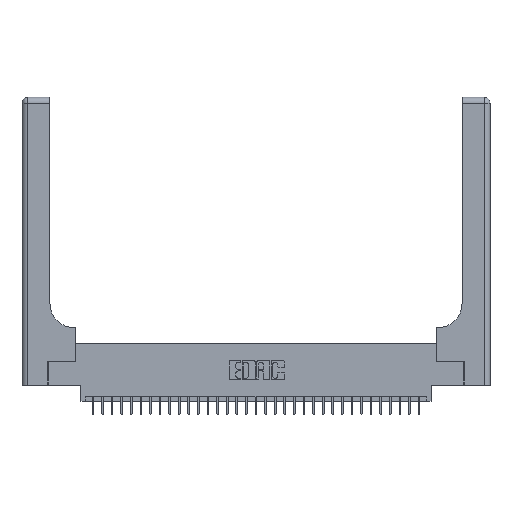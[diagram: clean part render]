
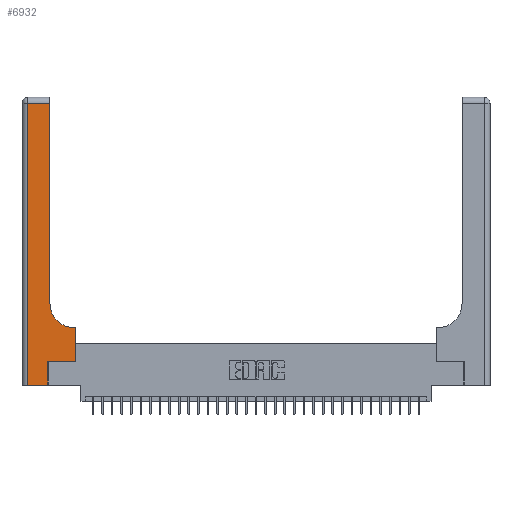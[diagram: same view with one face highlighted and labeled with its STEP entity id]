
A CAD part, top view. The second image highlights one B-rep face of the part: STEP entity #6932.
In plain terms, the highlighted planar face has unit normal (0, 0, 1).
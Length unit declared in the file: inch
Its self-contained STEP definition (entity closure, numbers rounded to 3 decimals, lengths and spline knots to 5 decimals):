
#358 = DIRECTION ( 'NONE',  ( 0., -1., 0. ) ) ;
#1039 = CARTESIAN_POINT ( 'NONE',  ( 0.269, 0.25, 0.37 ) ) ;
#2284 = VERTEX_POINT ( 'NONE', #19013 ) ;
#3089 = VERTEX_POINT ( 'NONE', #6242 ) ;
#4320 = LINE ( 'NONE', #20012, #7440 ) ;
#4754 = CARTESIAN_POINT ( 'NONE',  ( 0.2915, 0.85, 0.37 ) ) ;
#5016 = VERTEX_POINT ( 'NONE', #31382 ) ;
#5090 = DIRECTION ( 'NONE',  ( 1., 0., 0. ) ) ;
#5252 = VERTEX_POINT ( 'NONE', #15384 ) ;
#5537 = CARTESIAN_POINT ( 'NONE',  ( 0.06, 3., 0.37 ) ) ;
#6242 = CARTESIAN_POINT ( 'NONE',  ( 0.5585, 0.25, 0.37 ) ) ;
#6323 = CARTESIAN_POINT ( 'NONE',  ( 0.06, 0., 0.37 ) ) ;
#6932 = ADVANCED_FACE ( 'NONE', ( #25825 ), #18137, .F. ) ;
#7440 = VECTOR ( 'NONE', #17470, 39.37008 ) ;
#8544 = CARTESIAN_POINT ( 'NONE',  ( 0., 0., 0.37 ) ) ;
#8953 = LINE ( 'NONE', #32234, #21682 ) ;
#9383 = ORIENTED_EDGE ( 'NONE', *, *, #12861, .T. ) ;
#9558 = VECTOR ( 'NONE', #19587, 39.37008 ) ;
#9730 = EDGE_CURVE ( 'NONE', #16667, #9868, #18264, .T. ) ;
#9868 = VERTEX_POINT ( 'NONE', #16902 ) ;
#10740 = AXIS2_PLACEMENT_3D ( 'NONE', #18411, #31085, #5090 ) ;
#10835 = VECTOR ( 'NONE', #25276, 39.37008 ) ;
#11069 = VECTOR ( 'NONE', #23723, 39.37008 ) ;
#11149 = LINE ( 'NONE', #5537, #26065 ) ;
#11318 = CIRCLE ( 'NONE', #10740, 0.25 ) ;
#11717 = LINE ( 'NONE', #26955, #9558 ) ;
#12861 = EDGE_CURVE ( 'NONE', #22208, #5016, #16590, .T. ) ;
#15384 = CARTESIAN_POINT ( 'NONE',  ( 0.06, 2.94, 0.37 ) ) ;
#16389 = CARTESIAN_POINT ( 'NONE',  ( 0.2915, 3., 0.37 ) ) ;
#16590 = LINE ( 'NONE', #8544, #17673 ) ;
#16656 = DIRECTION ( 'NONE',  ( 0., 1., 0. ) ) ;
#16667 = VERTEX_POINT ( 'NONE', #4754 ) ;
#16744 = EDGE_CURVE ( 'NONE', #2284, #16667, #11318, .T. ) ;
#16902 = CARTESIAN_POINT ( 'NONE',  ( 0.2915, 2.94, 0.37 ) ) ;
#17432 = LINE ( 'NONE', #27864, #10835 ) ;
#17470 = DIRECTION ( 'NONE',  ( 0., 1., 0. ) ) ;
#17673 = VECTOR ( 'NONE', #19148, 39.37008 ) ;
#18137 = PLANE ( 'NONE',  #31477 ) ;
#18264 = LINE ( 'NONE', #16389, #11069 ) ;
#18411 = CARTESIAN_POINT ( 'NONE',  ( 0.5415, 0.85, 0.37 ) ) ;
#18789 = LINE ( 'NONE', #31796, #28362 ) ;
#18974 = EDGE_CURVE ( 'NONE', #5252, #22208, #11149, .T. ) ;
#19013 = CARTESIAN_POINT ( 'NONE',  ( 0.5415, 0.6, 0.37 ) ) ;
#19148 = DIRECTION ( 'NONE',  ( 1., 0., 0. ) ) ;
#19587 = DIRECTION ( 'NONE',  ( -1., 0., 0. ) ) ;
#20012 = CARTESIAN_POINT ( 'NONE',  ( 0.5585, 0.25, 0.37 ) ) ;
#20351 = ORIENTED_EDGE ( 'NONE', *, *, #29935, .T. ) ;
#20500 = ORIENTED_EDGE ( 'NONE', *, *, #9730, .T. ) ;
#21682 = VECTOR ( 'NONE', #16656, 39.37008 ) ;
#21769 = EDGE_CURVE ( 'NONE', #5016, #27297, #8953, .T. ) ;
#22053 = EDGE_CURVE ( 'NONE', #27297, #3089, #18789, .T. ) ;
#22208 = VERTEX_POINT ( 'NONE', #6323 ) ;
#23635 = CARTESIAN_POINT ( 'NONE',  ( 0.5585, 0.6, 0.37 ) ) ;
#23723 = DIRECTION ( 'NONE',  ( 0., 1., 0. ) ) ;
#24895 = ORIENTED_EDGE ( 'NONE', *, *, #32604, .T. ) ;
#25276 = DIRECTION ( 'NONE',  ( -1., 0., 0. ) ) ;
#25320 = DIRECTION ( 'NONE',  ( 0., 0., -1. ) ) ;
#25825 = FACE_OUTER_BOUND ( 'NONE', #26362, .T. ) ;
#25996 = CARTESIAN_POINT ( 'NONE',  ( 0., 3., 0.37 ) ) ;
#26065 = VECTOR ( 'NONE', #358, 39.37008 ) ;
#26362 = EDGE_LOOP ( 'NONE', ( #20500, #29959, #31094, #9383, #30911, #31027, #20351, #24895, #32363 ) ) ;
#26526 = EDGE_CURVE ( 'NONE', #9868, #5252, #11717, .T. ) ;
#26955 = CARTESIAN_POINT ( 'NONE',  ( 0., 2.94, 0.37 ) ) ;
#27297 = VERTEX_POINT ( 'NONE', #1039 ) ;
#27864 = CARTESIAN_POINT ( 'NONE',  ( 0.2915, 0.6, 0.37 ) ) ;
#28362 = VECTOR ( 'NONE', #29569, 39.37008 ) ;
#29569 = DIRECTION ( 'NONE',  ( 1., 0., 0. ) ) ;
#29611 = VERTEX_POINT ( 'NONE', #23635 ) ;
#29935 = EDGE_CURVE ( 'NONE', #3089, #29611, #4320, .T. ) ;
#29959 = ORIENTED_EDGE ( 'NONE', *, *, #26526, .T. ) ;
#30475 = DIRECTION ( 'NONE',  ( -1., 0., 0. ) ) ;
#30911 = ORIENTED_EDGE ( 'NONE', *, *, #21769, .T. ) ;
#31027 = ORIENTED_EDGE ( 'NONE', *, *, #22053, .T. ) ;
#31085 = DIRECTION ( 'NONE',  ( 0., 0., -1. ) ) ;
#31094 = ORIENTED_EDGE ( 'NONE', *, *, #18974, .T. ) ;
#31382 = CARTESIAN_POINT ( 'NONE',  ( 0.269, 0., 0.37 ) ) ;
#31477 = AXIS2_PLACEMENT_3D ( 'NONE', #25996, #25320, #30475 ) ;
#31796 = CARTESIAN_POINT ( 'NONE',  ( 0.269, 0.25, 0.37 ) ) ;
#32234 = CARTESIAN_POINT ( 'NONE',  ( 0.269, 0., 0.37 ) ) ;
#32363 = ORIENTED_EDGE ( 'NONE', *, *, #16744, .T. ) ;
#32604 = EDGE_CURVE ( 'NONE', #29611, #2284, #17432, .T. ) ;
